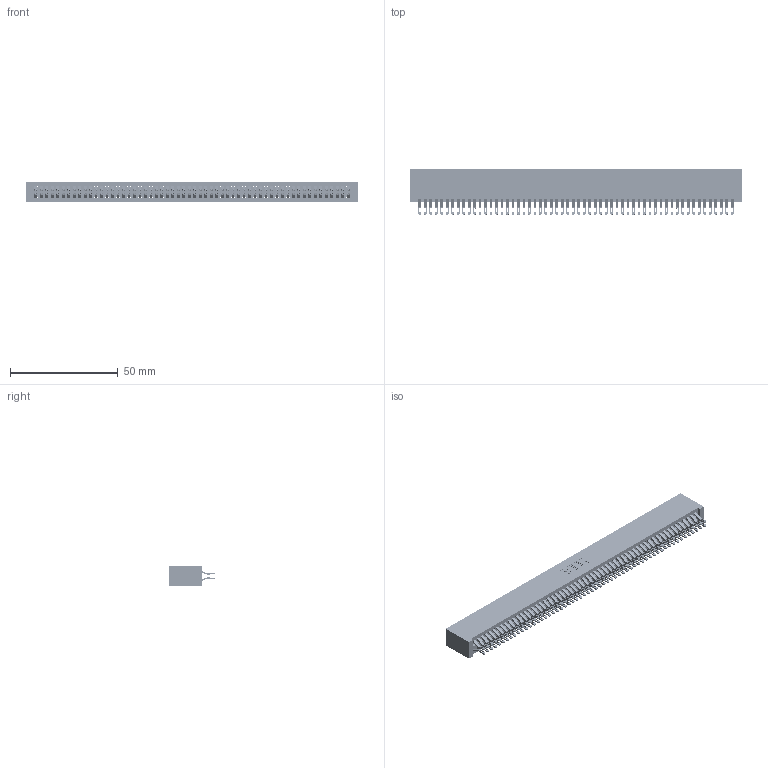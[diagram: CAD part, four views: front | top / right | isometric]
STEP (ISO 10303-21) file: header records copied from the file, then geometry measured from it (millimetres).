
FILE_DESCRIPTION (( 'STEP AP203' ), '1' );
FILE_NAME ('395-116-555-201.STEP', '2018-12-02T01:23:15', ( '' ), ( '' ), 'SwSTEP 2.0', 'SolidWorks 2016', '' );
FILE_SCHEMA (( 'CONFIG_CONTROL_DESIGN' ));
Length unit declared in the file: inch
Products named in the file (3): 345-292-001_555 Tail; 395-116-555-201; 345 Part_No Mounting Lugs
Assembly tree (117 placements, depth 2):
  395-116-555-201
    345 Part_No Mounting Lugs
    345-292-001_555 Tail  x116
Bounding box: 153.92 x 21.13 x 9.4 mm (x, y, z)
Volume: 16053.2 mm3; surface area: 25512.8 mm2
Topology: 117 solids, 117 shells, 6614 faces, 20849 edges, 13898 vertices
Faces by surface type: plane 3672, cylinder 2942
Entity records: 43403 total; most frequent: CARTESIAN_POINT 7294, ORIENTED_EDGE 7198, DIRECTION 6375, EDGE_CURVE 3599, VECTOR 3223, LINE 3223, VERTEX_POINT 2398, AXIS2_PLACEMENT_3D 1576
